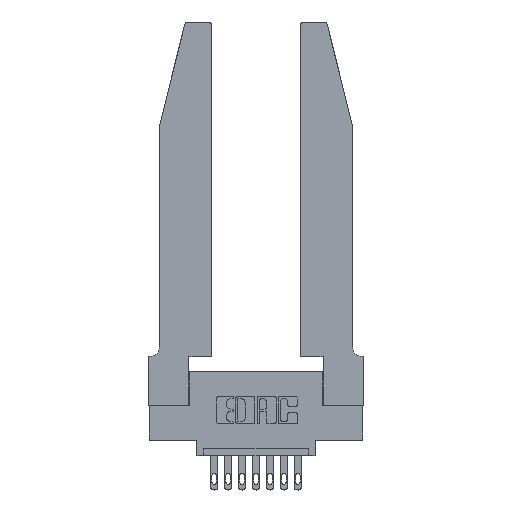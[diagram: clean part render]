
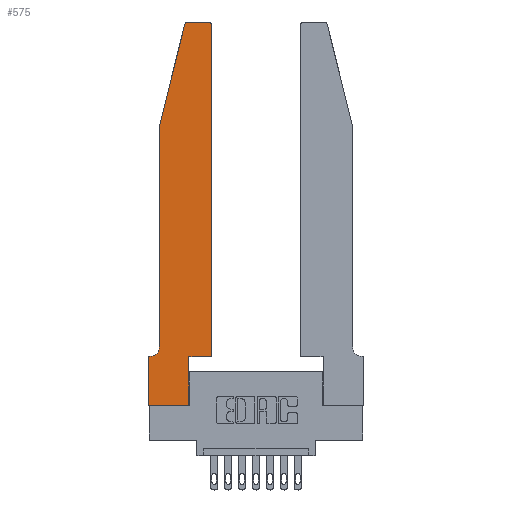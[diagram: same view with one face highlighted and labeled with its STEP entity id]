
A CAD part, top view. The second image highlights one B-rep face of the part: STEP entity #575.
In plain terms, the highlighted planar face has unit normal (0, 0, 1).
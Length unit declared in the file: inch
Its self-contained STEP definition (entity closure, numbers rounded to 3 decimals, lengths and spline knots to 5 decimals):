
#187 = VECTOR ( 'NONE', #7000, 39.37008 ) ;
#284 = DIRECTION ( 'NONE',  ( 1., 0., 0. ) ) ;
#564 = VECTOR ( 'NONE', #3813, 39.37008 ) ;
#575 = ADVANCED_FACE ( 'NONE', ( #5036 ), #5939, .T. ) ;
#600 = DIRECTION ( 'NONE',  ( 1., 0., 0. ) ) ;
#734 = DIRECTION ( 'NONE',  ( 1., 0., 0. ) ) ;
#852 = DIRECTION ( 'NONE',  ( 1., 0., 0. ) ) ;
#896 = LINE ( 'NONE', #3508, #5559 ) ;
#1039 = VERTEX_POINT ( 'NONE', #8213 ) ;
#1211 = ORIENTED_EDGE ( 'NONE', *, *, #2185, .T. ) ;
#1384 = DIRECTION ( 'NONE',  ( -0.239, -0.971, 0. ) ) ;
#1483 = ORIENTED_EDGE ( 'NONE', *, *, #11120, .T. ) ;
#1741 = CARTESIAN_POINT ( 'NONE',  ( 0.0755, 2., 0.37 ) ) ;
#1839 = DIRECTION ( 'NONE',  ( 0., 0., 1. ) ) ;
#2172 = ORIENTED_EDGE ( 'NONE', *, *, #7844, .T. ) ;
#2185 = EDGE_CURVE ( 'NONE', #1039, #8304, #6231, .T. ) ;
#2345 = CIRCLE ( 'NONE', #3365, 0.03 ) ;
#2347 = CARTESIAN_POINT ( 'NONE',  ( 0., 0.35, 0.37 ) ) ;
#2428 = LINE ( 'NONE', #6980, #14551 ) ;
#2584 = EDGE_LOOP ( 'NONE', ( #9496, #3482, #1211, #1483, #12397, #8971, #12276, #12537, #13037, #3963, #2172, #6530 ) ) ;
#2694 = DIRECTION ( 'NONE',  ( 0., 0., 1. ) ) ;
#2736 = CARTESIAN_POINT ( 'NONE',  ( 0.2865, 0.35, 0.37 ) ) ;
#2892 = VECTOR ( 'NONE', #6152, 39.37008 ) ;
#3289 = CIRCLE ( 'NONE', #8372, 0.07 ) ;
#3365 = AXIS2_PLACEMENT_3D ( 'NONE', #8590, #1839, #734 ) ;
#3387 = DIRECTION ( 'NONE',  ( -1., 0., 0. ) ) ;
#3482 = ORIENTED_EDGE ( 'NONE', *, *, #11861, .T. ) ;
#3508 = CARTESIAN_POINT ( 'NONE',  ( 0., 0., 0.37 ) ) ;
#3517 = CARTESIAN_POINT ( 'NONE',  ( 0.0755, 2., 0.37 ) ) ;
#3547 = VERTEX_POINT ( 'NONE', #12075 ) ;
#3716 = AXIS2_PLACEMENT_3D ( 'NONE', #13140, #7451, #600 ) ;
#3802 = CARTESIAN_POINT ( 'NONE',  ( 0., 0., 0.37 ) ) ;
#3813 = DIRECTION ( 'NONE',  ( 0., -1., 0. ) ) ;
#3897 = VECTOR ( 'NONE', #1384, 39.37008 ) ;
#3963 = ORIENTED_EDGE ( 'NONE', *, *, #7372, .T. ) ;
#4165 = LINE ( 'NONE', #3802, #7381 ) ;
#4729 = EDGE_CURVE ( 'NONE', #10334, #10060, #2428, .T. ) ;
#5036 = FACE_OUTER_BOUND ( 'NONE', #2584, .T. ) ;
#5130 = CARTESIAN_POINT ( 'NONE',  ( 0., 0., 0.37 ) ) ;
#5190 = CIRCLE ( 'NONE', #3716, 0.03 ) ;
#5407 = VERTEX_POINT ( 'NONE', #13027 ) ;
#5408 = DIRECTION ( 'NONE',  ( 0., 1., 0. ) ) ;
#5485 = EDGE_CURVE ( 'NONE', #6936, #10334, #3289, .T. ) ;
#5512 = CARTESIAN_POINT ( 'NONE',  ( 0.4505, 0.35, 0.37 ) ) ;
#5559 = VECTOR ( 'NONE', #12445, 39.37008 ) ;
#5864 = VERTEX_POINT ( 'NONE', #9546 ) ;
#5939 = PLANE ( 'NONE',  #10720 ) ;
#6102 = DIRECTION ( 'NONE',  ( 1., 0., 0. ) ) ;
#6152 = DIRECTION ( 'NONE',  ( 0., 1., 0. ) ) ;
#6231 = LINE ( 'NONE', #3517, #3897 ) ;
#6294 = LINE ( 'NONE', #12898, #564 ) ;
#6530 = ORIENTED_EDGE ( 'NONE', *, *, #8736, .T. ) ;
#6642 = VERTEX_POINT ( 'NONE', #12715 ) ;
#6936 = VERTEX_POINT ( 'NONE', #11538 ) ;
#6980 = CARTESIAN_POINT ( 'NONE',  ( 0.0755, 0.35, 0.37 ) ) ;
#7000 = DIRECTION ( 'NONE',  ( -1., 0., 0. ) ) ;
#7001 = LINE ( 'NONE', #12703, #187 ) ;
#7068 = EDGE_CURVE ( 'NONE', #9150, #14790, #4165, .T. ) ;
#7372 = EDGE_CURVE ( 'NONE', #12419, #5407, #8436, .T. ) ;
#7381 = VECTOR ( 'NONE', #6102, 39.37008 ) ;
#7451 = DIRECTION ( 'NONE',  ( 0., 0., 1. ) ) ;
#7844 = EDGE_CURVE ( 'NONE', #5407, #6642, #10934, .T. ) ;
#7942 = EDGE_CURVE ( 'NONE', #5864, #3547, #7001, .T. ) ;
#8213 = CARTESIAN_POINT ( 'NONE',  ( 0.25487, 2.72718, 0.37 ) ) ;
#8304 = VERTEX_POINT ( 'NONE', #1741 ) ;
#8372 = AXIS2_PLACEMENT_3D ( 'NONE', #14273, #8628, #13175 ) ;
#8436 = LINE ( 'NONE', #5512, #10757 ) ;
#8590 = CARTESIAN_POINT ( 'NONE',  ( 0.284, 2.72, 0.37 ) ) ;
#8628 = DIRECTION ( 'NONE',  ( 0., 0., -1. ) ) ;
#8736 = EDGE_CURVE ( 'NONE', #6642, #5864, #5190, .T. ) ;
#8952 = LINE ( 'NONE', #10793, #2892 ) ;
#8971 = ORIENTED_EDGE ( 'NONE', *, *, #4729, .T. ) ;
#9150 = VERTEX_POINT ( 'NONE', #5130 ) ;
#9454 = CARTESIAN_POINT ( 'NONE',  ( 0., 0.35, 0.37 ) ) ;
#9496 = ORIENTED_EDGE ( 'NONE', *, *, #7942, .T. ) ;
#9546 = CARTESIAN_POINT ( 'NONE',  ( 0.4205, 2.75, 0.37 ) ) ;
#10060 = VERTEX_POINT ( 'NONE', #9454 ) ;
#10334 = VERTEX_POINT ( 'NONE', #12533 ) ;
#10720 = AXIS2_PLACEMENT_3D ( 'NONE', #2347, #2694, #284 ) ;
#10757 = VECTOR ( 'NONE', #852, 39.37008 ) ;
#10793 = CARTESIAN_POINT ( 'NONE',  ( 0.2865, 0.35, 0.37 ) ) ;
#10934 = LINE ( 'NONE', #11286, #11625 ) ;
#11120 = EDGE_CURVE ( 'NONE', #8304, #6936, #6294, .T. ) ;
#11286 = CARTESIAN_POINT ( 'NONE',  ( 0.4505, 0.35, 0.37 ) ) ;
#11415 = EDGE_CURVE ( 'NONE', #10060, #9150, #896, .T. ) ;
#11538 = CARTESIAN_POINT ( 'NONE',  ( 0.0755, 0.42, 0.37 ) ) ;
#11625 = VECTOR ( 'NONE', #5408, 39.37008 ) ;
#11746 = EDGE_CURVE ( 'NONE', #14790, #12419, #8952, .T. ) ;
#11861 = EDGE_CURVE ( 'NONE', #3547, #1039, #2345, .T. ) ;
#12075 = CARTESIAN_POINT ( 'NONE',  ( 0.284, 2.75, 0.37 ) ) ;
#12276 = ORIENTED_EDGE ( 'NONE', *, *, #11415, .T. ) ;
#12397 = ORIENTED_EDGE ( 'NONE', *, *, #5485, .T. ) ;
#12419 = VERTEX_POINT ( 'NONE', #2736 ) ;
#12445 = DIRECTION ( 'NONE',  ( 0., -1., 0. ) ) ;
#12533 = CARTESIAN_POINT ( 'NONE',  ( 0.0055, 0.35, 0.37 ) ) ;
#12537 = ORIENTED_EDGE ( 'NONE', *, *, #7068, .T. ) ;
#12703 = CARTESIAN_POINT ( 'NONE',  ( 0.2605, 2.75, 0.37 ) ) ;
#12715 = CARTESIAN_POINT ( 'NONE',  ( 0.4505, 2.72, 0.37 ) ) ;
#12898 = CARTESIAN_POINT ( 'NONE',  ( 0.0755, 2., 0.37 ) ) ;
#13027 = CARTESIAN_POINT ( 'NONE',  ( 0.4505, 0.35, 0.37 ) ) ;
#13037 = ORIENTED_EDGE ( 'NONE', *, *, #11746, .T. ) ;
#13140 = CARTESIAN_POINT ( 'NONE',  ( 0.4205, 2.72, 0.37 ) ) ;
#13175 = DIRECTION ( 'NONE',  ( -1., 0., 0. ) ) ;
#14273 = CARTESIAN_POINT ( 'NONE',  ( 0.0055, 0.42, 0.37 ) ) ;
#14551 = VECTOR ( 'NONE', #3387, 39.37008 ) ;
#14623 = CARTESIAN_POINT ( 'NONE',  ( 0.2865, 0., 0.37 ) ) ;
#14790 = VERTEX_POINT ( 'NONE', #14623 ) ;
